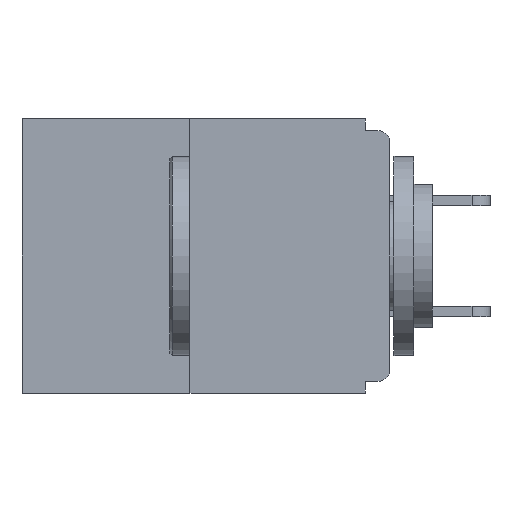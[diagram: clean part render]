
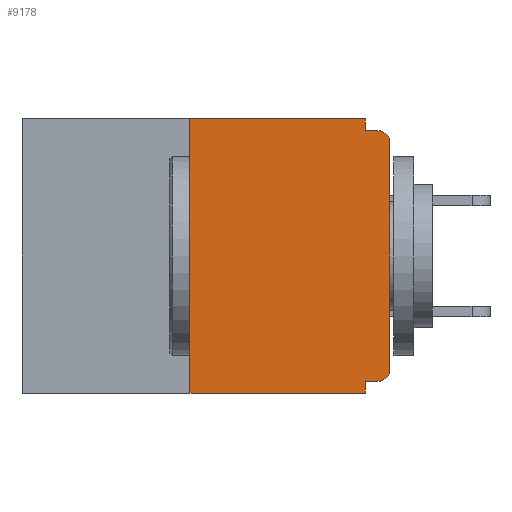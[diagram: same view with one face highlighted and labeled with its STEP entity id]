
A CAD part, left-side view. The second image highlights one B-rep face of the part: STEP entity #9178.
In plain terms, the highlighted planar face has unit normal (-1, 0, 0).
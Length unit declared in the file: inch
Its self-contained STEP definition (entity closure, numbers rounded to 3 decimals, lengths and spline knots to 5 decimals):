
#29 = CARTESIAN_POINT ( 'NONE',  ( 0., 0., -0.015 ) ) ;
#130 = LINE ( 'NONE', #7690, #23282 ) ;
#310 = CARTESIAN_POINT ( 'NONE',  ( 0., 0.031, -0.343 ) ) ;
#1222 = EDGE_CURVE ( 'NONE', #21746, #23497, #13030, .T. ) ;
#1781 = EDGE_CURVE ( 'NONE', #18973, #8208, #130, .T. ) ;
#1951 = ORIENTED_EDGE ( 'NONE', *, *, #6694, .T. ) ;
#2402 = LINE ( 'NONE', #21412, #23528 ) ;
#2476 = ORIENTED_EDGE ( 'NONE', *, *, #1781, .F. ) ;
#2750 = LINE ( 'NONE', #8529, #21529 ) ;
#3341 = DIRECTION ( 'NONE',  ( 0., 0., 1. ) ) ;
#3813 = EDGE_CURVE ( 'NONE', #12497, #27935, #19409, .T. ) ;
#4271 = CIRCLE ( 'NONE', #14747, 0.015 ) ;
#4485 = VERTEX_POINT ( 'NONE', #9016 ) ;
#4542 = CARTESIAN_POINT ( 'NONE',  ( 0., 0.031, -0.343 ) ) ;
#5082 = CARTESIAN_POINT ( 'NONE',  ( 0., 0.015, -0.328 ) ) ;
#5463 = DIRECTION ( 'NONE',  ( 0., 0., -1. ) ) ;
#6694 = EDGE_CURVE ( 'NONE', #15039, #4485, #4271, .T. ) ;
#7083 = DIRECTION ( 'NONE',  ( 0., 1., 0. ) ) ;
#7365 = EDGE_CURVE ( 'NONE', #8270, #8951, #24649, .T. ) ;
#7371 = DIRECTION ( 'NONE',  ( -1., 0., 0. ) ) ;
#7690 = CARTESIAN_POINT ( 'NONE',  ( 0., 0.031, 0. ) ) ;
#8027 = LINE ( 'NONE', #9191, #10081 ) ;
#8208 = VERTEX_POINT ( 'NONE', #14508 ) ;
#8242 = EDGE_LOOP ( 'NONE', ( #14433, #25113, #27719, #20222, #17517, #1951, #16140, #24812, #16672, #2476 ) ) ;
#8270 = VERTEX_POINT ( 'NONE', #18930 ) ;
#8529 = CARTESIAN_POINT ( 'NONE',  ( 0., 0., -0.328 ) ) ;
#8951 = VERTEX_POINT ( 'NONE', #4542 ) ;
#9016 = CARTESIAN_POINT ( 'NONE',  ( 0., 0., -0.313 ) ) ;
#9166 = CARTESIAN_POINT ( 'NONE',  ( 0., 0., 0. ) ) ;
#9178 = ADVANCED_FACE ( 'NONE', ( #13377 ), #19186, .F. ) ;
#9191 = CARTESIAN_POINT ( 'NONE',  ( 0., 0.46, -0.343 ) ) ;
#9310 = EDGE_CURVE ( 'NONE', #15039, #8270, #2750, .T. ) ;
#10081 = VECTOR ( 'NONE', #11412, 39.37008 ) ;
#10184 = DIRECTION ( 'NONE',  ( 0., 0., -1. ) ) ;
#10268 = DIRECTION ( 'NONE',  ( 0., 0., -1. ) ) ;
#10344 = VECTOR ( 'NONE', #20095, 39.37008 ) ;
#10423 = DIRECTION ( 'NONE',  ( 0., -1., 0. ) ) ;
#10904 = CARTESIAN_POINT ( 'NONE',  ( 0., 0.25, 0. ) ) ;
#11220 = DIRECTION ( 'NONE',  ( -1., 0., 0. ) ) ;
#11412 = DIRECTION ( 'NONE',  ( 0., -1., 0. ) ) ;
#12497 = VERTEX_POINT ( 'NONE', #18597 ) ;
#13030 = CIRCLE ( 'NONE', #21171, 0.015 ) ;
#13377 = FACE_OUTER_BOUND ( 'NONE', #8242, .T. ) ;
#13495 = CARTESIAN_POINT ( 'NONE',  ( 0., 0.031, 0. ) ) ;
#13562 = DIRECTION ( 'NONE',  ( 0., 0., -1. ) ) ;
#14433 = ORIENTED_EDGE ( 'NONE', *, *, #24051, .F. ) ;
#14508 = CARTESIAN_POINT ( 'NONE',  ( 0., 0.031, -0.015 ) ) ;
#14747 = AXIS2_PLACEMENT_3D ( 'NONE', #15489, #11220, #17747 ) ;
#15039 = VERTEX_POINT ( 'NONE', #5082 ) ;
#15489 = CARTESIAN_POINT ( 'NONE',  ( 0., 0.015, -0.313 ) ) ;
#16140 = ORIENTED_EDGE ( 'NONE', *, *, #21962, .T. ) ;
#16420 = CARTESIAN_POINT ( 'NONE',  ( 0., 0.25, 0. ) ) ;
#16672 = ORIENTED_EDGE ( 'NONE', *, *, #23418, .F. ) ;
#16939 = CARTESIAN_POINT ( 'NONE',  ( 0., 0.46, 0. ) ) ;
#17465 = CARTESIAN_POINT ( 'NONE',  ( 0., 0.015, -0.015 ) ) ;
#17517 = ORIENTED_EDGE ( 'NONE', *, *, #9310, .F. ) ;
#17747 = DIRECTION ( 'NONE',  ( 0., 0., -1. ) ) ;
#18486 = CARTESIAN_POINT ( 'NONE',  ( 0., 0.015, -0.03 ) ) ;
#18597 = CARTESIAN_POINT ( 'NONE',  ( 0., 0.25, -0.343 ) ) ;
#18930 = CARTESIAN_POINT ( 'NONE',  ( 0., 0.031, -0.328 ) ) ;
#18973 = VERTEX_POINT ( 'NONE', #13495 ) ;
#19080 = VECTOR ( 'NONE', #3341, 39.37008 ) ;
#19186 = PLANE ( 'NONE',  #21679 ) ;
#19409 = LINE ( 'NONE', #16420, #19080 ) ;
#19760 = VECTOR ( 'NONE', #10423, 39.37008 ) ;
#20095 = DIRECTION ( 'NONE',  ( 0., 0., 1. ) ) ;
#20222 = ORIENTED_EDGE ( 'NONE', *, *, #7365, .F. ) ;
#20436 = EDGE_CURVE ( 'NONE', #12497, #8951, #8027, .T. ) ;
#21171 = AXIS2_PLACEMENT_3D ( 'NONE', #18486, #7371, #5463 ) ;
#21412 = CARTESIAN_POINT ( 'NONE',  ( 0., 0.46, 0. ) ) ;
#21529 = VECTOR ( 'NONE', #7083, 39.37008 ) ;
#21679 = AXIS2_PLACEMENT_3D ( 'NONE', #16939, #25542, #10268 ) ;
#21746 = VERTEX_POINT ( 'NONE', #27273 ) ;
#21962 = EDGE_CURVE ( 'NONE', #4485, #21746, #27680, .T. ) ;
#23282 = VECTOR ( 'NONE', #10184, 39.37008 ) ;
#23418 = EDGE_CURVE ( 'NONE', #8208, #23497, #25543, .T. ) ;
#23497 = VERTEX_POINT ( 'NONE', #17465 ) ;
#23528 = VECTOR ( 'NONE', #27940, 39.37008 ) ;
#24051 = EDGE_CURVE ( 'NONE', #27935, #18973, #2402, .T. ) ;
#24649 = LINE ( 'NONE', #310, #26335 ) ;
#24812 = ORIENTED_EDGE ( 'NONE', *, *, #1222, .T. ) ;
#25113 = ORIENTED_EDGE ( 'NONE', *, *, #3813, .F. ) ;
#25542 = DIRECTION ( 'NONE',  ( 1., 0., 0. ) ) ;
#25543 = LINE ( 'NONE', #29, #19760 ) ;
#26335 = VECTOR ( 'NONE', #13562, 39.37008 ) ;
#27273 = CARTESIAN_POINT ( 'NONE',  ( 0., 0., -0.03 ) ) ;
#27680 = LINE ( 'NONE', #9166, #10344 ) ;
#27719 = ORIENTED_EDGE ( 'NONE', *, *, #20436, .T. ) ;
#27935 = VERTEX_POINT ( 'NONE', #10904 ) ;
#27940 = DIRECTION ( 'NONE',  ( 0., -1., 0. ) ) ;
